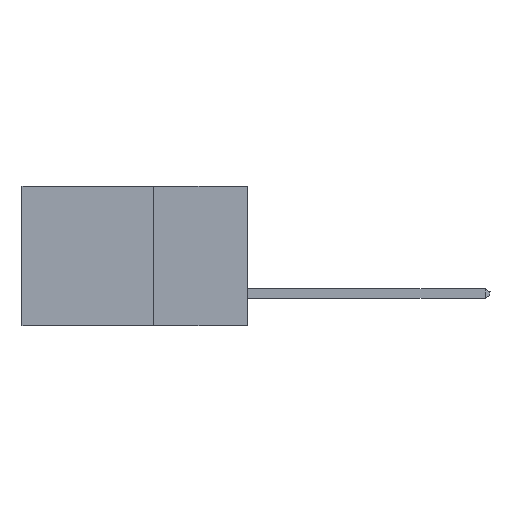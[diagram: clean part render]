
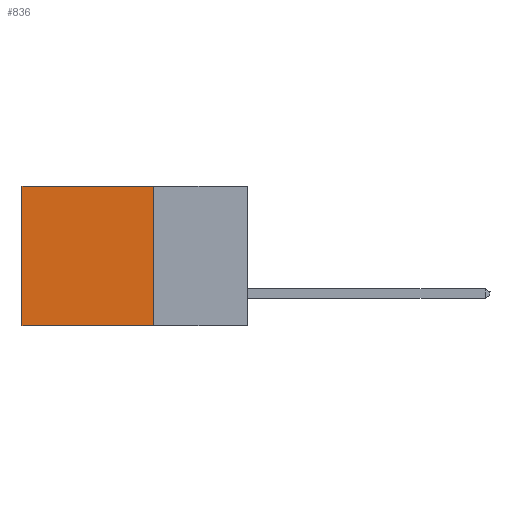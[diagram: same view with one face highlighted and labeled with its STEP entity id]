
A CAD part, left-side view. The second image highlights one B-rep face of the part: STEP entity #836.
In plain terms, the highlighted planar face has unit normal (-1, 0, 0).
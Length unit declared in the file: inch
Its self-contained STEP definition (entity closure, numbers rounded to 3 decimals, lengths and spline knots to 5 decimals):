
#149 = CARTESIAN_POINT ( 'NONE',  ( 0.2615, 0.6, 0. ) ) ;
#328 = DIRECTION ( 'NONE',  ( 0., 1., 0. ) ) ;
#836 = ADVANCED_FACE ( 'NONE', ( #21031 ), #7092, .F. ) ;
#1007 = ORIENTED_EDGE ( 'NONE', *, *, #1396, .F. ) ;
#1143 = CARTESIAN_POINT ( 'NONE',  ( 0.2615, 0.25, -0.37 ) ) ;
#1396 = EDGE_CURVE ( 'NONE', #13474, #2306, #5528, .T. ) ;
#1430 = VERTEX_POINT ( 'NONE', #14592 ) ;
#1585 = VECTOR ( 'NONE', #328, 39.37008 ) ;
#1864 = EDGE_LOOP ( 'NONE', ( #17119, #1007, #15226, #5788 ) ) ;
#1941 = CARTESIAN_POINT ( 'NONE',  ( 0.2615, 0.25, -0.37 ) ) ;
#2306 = VERTEX_POINT ( 'NONE', #9108 ) ;
#2318 = CARTESIAN_POINT ( 'NONE',  ( 0.2615, 0.25, -0.37 ) ) ;
#2430 = LINE ( 'NONE', #20348, #7421 ) ;
#5308 = CARTESIAN_POINT ( 'NONE',  ( 0.2615, 0.6, -0.37 ) ) ;
#5528 = LINE ( 'NONE', #5644, #1585 ) ;
#5644 = CARTESIAN_POINT ( 'NONE',  ( 0.2615, 0.25, -0.37 ) ) ;
#5788 = ORIENTED_EDGE ( 'NONE', *, *, #13132, .T. ) ;
#6851 = EDGE_CURVE ( 'NONE', #9969, #2306, #10606, .T. ) ;
#7092 = PLANE ( 'NONE',  #22323 ) ;
#7421 = VECTOR ( 'NONE', #17152, 39.37008 ) ;
#7712 = EDGE_CURVE ( 'NONE', #1430, #13474, #10939, .T. ) ;
#9108 = CARTESIAN_POINT ( 'NONE',  ( 0.2615, 0.6, -0.37 ) ) ;
#9969 = VERTEX_POINT ( 'NONE', #149 ) ;
#10606 = LINE ( 'NONE', #5308, #10822 ) ;
#10822 = VECTOR ( 'NONE', #12493, 39.37008 ) ;
#10939 = LINE ( 'NONE', #2318, #14880 ) ;
#12493 = DIRECTION ( 'NONE',  ( 0., 0., -1. ) ) ;
#13050 = DIRECTION ( 'NONE',  ( 0., 0., -1. ) ) ;
#13132 = EDGE_CURVE ( 'NONE', #1430, #9969, #2430, .T. ) ;
#13474 = VERTEX_POINT ( 'NONE', #1941 ) ;
#14285 = DIRECTION ( 'NONE',  ( 0., 0., -1. ) ) ;
#14592 = CARTESIAN_POINT ( 'NONE',  ( 0.2615, 0.25, 0. ) ) ;
#14880 = VECTOR ( 'NONE', #13050, 39.37008 ) ;
#15226 = ORIENTED_EDGE ( 'NONE', *, *, #7712, .F. ) ;
#16155 = DIRECTION ( 'NONE',  ( 1., 0., 0. ) ) ;
#17119 = ORIENTED_EDGE ( 'NONE', *, *, #6851, .T. ) ;
#17152 = DIRECTION ( 'NONE',  ( 0., 1., 0. ) ) ;
#20348 = CARTESIAN_POINT ( 'NONE',  ( 0.2615, 0.25, 0. ) ) ;
#21031 = FACE_OUTER_BOUND ( 'NONE', #1864, .T. ) ;
#22323 = AXIS2_PLACEMENT_3D ( 'NONE', #1143, #16155, #14285 ) ;
